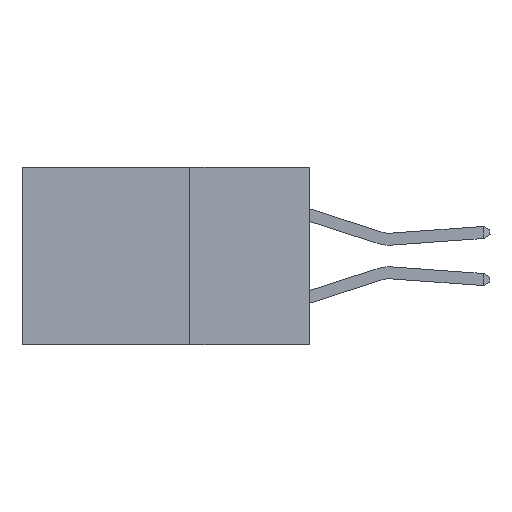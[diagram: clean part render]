
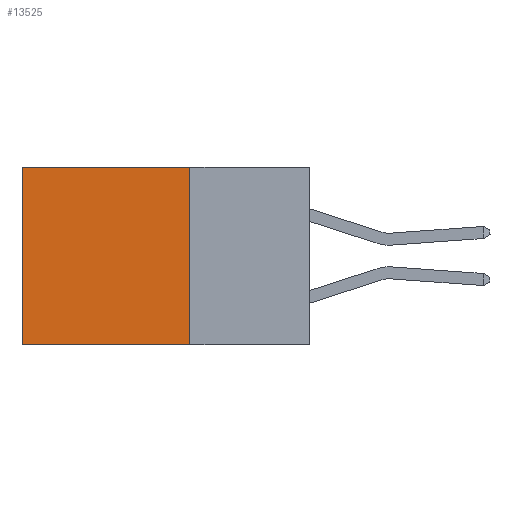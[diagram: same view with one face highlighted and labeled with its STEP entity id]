
A CAD part, left-side view. The second image highlights one B-rep face of the part: STEP entity #13525.
In plain terms, the highlighted planar face has unit normal (-1, 0, 0).
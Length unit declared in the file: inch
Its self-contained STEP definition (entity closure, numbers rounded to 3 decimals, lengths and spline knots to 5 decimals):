
#78 = EDGE_CURVE ( 'NONE', #7157, #8827, #14078, .T. ) ;
#184 = EDGE_CURVE ( 'NONE', #9898, #10182, #10613, .T. ) ;
#199 = ORIENTED_EDGE ( 'NONE', *, *, #78, .T. ) ;
#230 = CARTESIAN_POINT ( 'NONE',  ( 0.2615, 0.6, 0. ) ) ;
#320 = CARTESIAN_POINT ( 'NONE',  ( 0.2615, 0.6, -0.37 ) ) ;
#1128 = PLANE ( 'NONE',  #7844 ) ;
#1792 = LINE ( 'NONE', #7708, #9782 ) ;
#3787 = CARTESIAN_POINT ( 'NONE',  ( 0.2615, 0.25, 0. ) ) ;
#5265 = CARTESIAN_POINT ( 'NONE',  ( 0.2615, 0.25, -0.37 ) ) ;
#5411 = ORIENTED_EDGE ( 'NONE', *, *, #16170, .T. ) ;
#5861 = CARTESIAN_POINT ( 'NONE',  ( 0.2615, 0.25, 0. ) ) ;
#6159 = LINE ( 'NONE', #13013, #7244 ) ;
#6230 = CARTESIAN_POINT ( 'NONE',  ( 0.2615, 0.25, -0.37 ) ) ;
#7157 = VERTEX_POINT ( 'NONE', #3787 ) ;
#7244 = VECTOR ( 'NONE', #7621, 39.37008 ) ;
#7621 = DIRECTION ( 'NONE',  ( 0., 0., -1. ) ) ;
#7708 = CARTESIAN_POINT ( 'NONE',  ( 0.2615, 0.6, -0.37 ) ) ;
#7844 = AXIS2_PLACEMENT_3D ( 'NONE', #12088, #16287, #16099 ) ;
#8827 = VERTEX_POINT ( 'NONE', #230 ) ;
#9149 = ORIENTED_EDGE ( 'NONE', *, *, #14583, .F. ) ;
#9782 = VECTOR ( 'NONE', #13286, 39.37008 ) ;
#9898 = VERTEX_POINT ( 'NONE', #5265 ) ;
#10182 = VERTEX_POINT ( 'NONE', #320 ) ;
#10302 = VECTOR ( 'NONE', #12723, 39.37008 ) ;
#10613 = LINE ( 'NONE', #6230, #15260 ) ;
#10722 = FACE_OUTER_BOUND ( 'NONE', #13537, .T. ) ;
#11989 = DIRECTION ( 'NONE',  ( 0., 1., 0. ) ) ;
#12088 = CARTESIAN_POINT ( 'NONE',  ( 0.2615, 0.25, -0.37 ) ) ;
#12723 = DIRECTION ( 'NONE',  ( 0., 1., 0. ) ) ;
#13013 = CARTESIAN_POINT ( 'NONE',  ( 0.2615, 0.25, -0.37 ) ) ;
#13286 = DIRECTION ( 'NONE',  ( 0., 0., -1. ) ) ;
#13525 = ADVANCED_FACE ( 'NONE', ( #10722 ), #1128, .F. ) ;
#13537 = EDGE_LOOP ( 'NONE', ( #5411, #17405, #9149, #199 ) ) ;
#14078 = LINE ( 'NONE', #5861, #10302 ) ;
#14583 = EDGE_CURVE ( 'NONE', #7157, #9898, #6159, .T. ) ;
#15260 = VECTOR ( 'NONE', #11989, 39.37008 ) ;
#16099 = DIRECTION ( 'NONE',  ( 0., 0., -1. ) ) ;
#16170 = EDGE_CURVE ( 'NONE', #8827, #10182, #1792, .T. ) ;
#16287 = DIRECTION ( 'NONE',  ( 1., 0., 0. ) ) ;
#17405 = ORIENTED_EDGE ( 'NONE', *, *, #184, .F. ) ;
